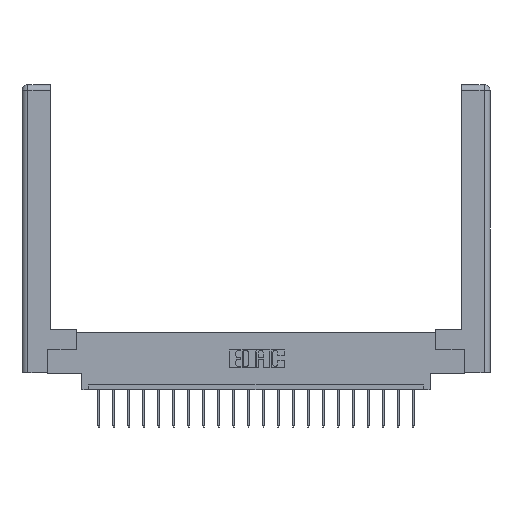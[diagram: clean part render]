
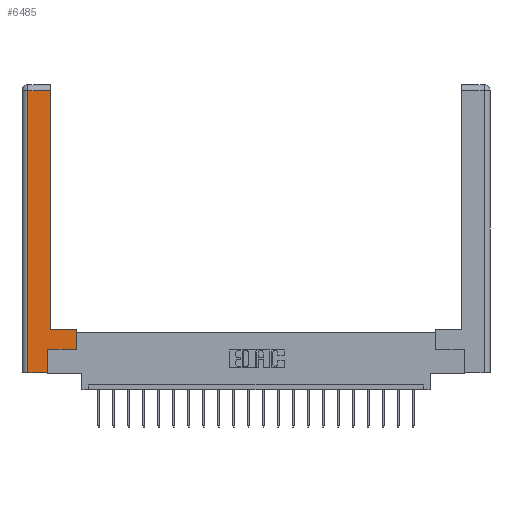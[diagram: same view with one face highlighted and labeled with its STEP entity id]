
A CAD part, top view. The second image highlights one B-rep face of the part: STEP entity #6485.
In plain terms, the highlighted planar face has unit normal (0, 0, 1).
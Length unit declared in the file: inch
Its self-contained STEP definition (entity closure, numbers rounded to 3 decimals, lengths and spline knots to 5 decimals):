
#283 = VERTEX_POINT ( 'NONE', #10952 ) ;
#550 = CARTESIAN_POINT ( 'NONE',  ( 0.0615, 0., 0. ) ) ;
#980 = CARTESIAN_POINT ( 'NONE',  ( 0.565, 0.45, 0. ) ) ;
#1034 = EDGE_CURVE ( 'NONE', #2559, #15257, #3700, .T. ) ;
#1696 = ORIENTED_EDGE ( 'NONE', *, *, #19010, .T. ) ;
#1902 = EDGE_CURVE ( 'NONE', #12222, #6692, #17325, .T. ) ;
#2559 = VERTEX_POINT ( 'NONE', #18048 ) ;
#2889 = VECTOR ( 'NONE', #8444, 39.37008 ) ;
#3086 = DIRECTION ( 'NONE',  ( 0., 0., -1. ) ) ;
#3100 = CARTESIAN_POINT ( 'NONE',  ( 0.295, 0.45, 0. ) ) ;
#3181 = CARTESIAN_POINT ( 'NONE',  ( 0.295, 2.94, 0. ) ) ;
#3634 = FACE_OUTER_BOUND ( 'NONE', #5807, .T. ) ;
#3700 = LINE ( 'NONE', #15891, #17621 ) ;
#4054 = ORIENTED_EDGE ( 'NONE', *, *, #15213, .T. ) ;
#4450 = VECTOR ( 'NONE', #7974, 39.37008 ) ;
#4547 = CARTESIAN_POINT ( 'NONE',  ( 0.565, 0.245, 0. ) ) ;
#5807 = EDGE_LOOP ( 'NONE', ( #4054, #19135, #12590, #9939, #9728, #1696, #17788, #13337 ) ) ;
#6485 = ADVANCED_FACE ( 'NONE', ( #3634 ), #11439, .F. ) ;
#6692 = VERTEX_POINT ( 'NONE', #550 ) ;
#7974 = DIRECTION ( 'NONE',  ( 1., 0., 0. ) ) ;
#8112 = VERTEX_POINT ( 'NONE', #3100 ) ;
#8289 = LINE ( 'NONE', #17586, #18035 ) ;
#8444 = DIRECTION ( 'NONE',  ( 0., -1., 0. ) ) ;
#8876 = LINE ( 'NONE', #4547, #4450 ) ;
#9175 = EDGE_CURVE ( 'NONE', #13286, #283, #17426, .T. ) ;
#9404 = VECTOR ( 'NONE', #20173, 39.37008 ) ;
#9728 = ORIENTED_EDGE ( 'NONE', *, *, #1034, .T. ) ;
#9811 = DIRECTION ( 'NONE',  ( -1., 0., 0. ) ) ;
#9939 = ORIENTED_EDGE ( 'NONE', *, *, #19619, .T. ) ;
#10952 = CARTESIAN_POINT ( 'NONE',  ( 0.565, 0.45, 0. ) ) ;
#11193 = DIRECTION ( 'NONE',  ( 0., 1., 0. ) ) ;
#11387 = DIRECTION ( 'NONE',  ( -1., 0., 0. ) ) ;
#11439 = PLANE ( 'NONE',  #18159 ) ;
#12222 = VERTEX_POINT ( 'NONE', #15771 ) ;
#12590 = ORIENTED_EDGE ( 'NONE', *, *, #1902, .T. ) ;
#12798 = LINE ( 'NONE', #13486, #9404 ) ;
#13012 = EDGE_CURVE ( 'NONE', #13181, #12222, #20869, .T. ) ;
#13027 = CARTESIAN_POINT ( 'NONE',  ( 0., 0., 0. ) ) ;
#13181 = VERTEX_POINT ( 'NONE', #3181 ) ;
#13286 = VERTEX_POINT ( 'NONE', #18941 ) ;
#13337 = ORIENTED_EDGE ( 'NONE', *, *, #15268, .T. ) ;
#13486 = CARTESIAN_POINT ( 'NONE',  ( 0.265, 0., 0. ) ) ;
#14072 = LINE ( 'NONE', #14487, #21687 ) ;
#14261 = DIRECTION ( 'NONE',  ( -1., 0., 0. ) ) ;
#14487 = CARTESIAN_POINT ( 'NONE',  ( 0.295, 3., 0. ) ) ;
#14568 = CARTESIAN_POINT ( 'NONE',  ( 0.265, 0.245, 0. ) ) ;
#15208 = CARTESIAN_POINT ( 'NONE',  ( 0.0615, 2.94, 0. ) ) ;
#15213 = EDGE_CURVE ( 'NONE', #8112, #13181, #14072, .T. ) ;
#15257 = VERTEX_POINT ( 'NONE', #14568 ) ;
#15268 = EDGE_CURVE ( 'NONE', #283, #8112, #8289, .T. ) ;
#15737 = DIRECTION ( 'NONE',  ( 0., 1., 0. ) ) ;
#15755 = CARTESIAN_POINT ( 'NONE',  ( 0.0615, 0., 0. ) ) ;
#15771 = CARTESIAN_POINT ( 'NONE',  ( 0.0615, 2.94, 0. ) ) ;
#15891 = CARTESIAN_POINT ( 'NONE',  ( 0.265, 0.245, 0. ) ) ;
#16892 = VECTOR ( 'NONE', #15737, 39.37008 ) ;
#17325 = LINE ( 'NONE', #15755, #2889 ) ;
#17426 = LINE ( 'NONE', #980, #16892 ) ;
#17586 = CARTESIAN_POINT ( 'NONE',  ( 0.295, 0.45, 0. ) ) ;
#17621 = VECTOR ( 'NONE', #19348, 39.37008 ) ;
#17788 = ORIENTED_EDGE ( 'NONE', *, *, #9175, .T. ) ;
#18035 = VECTOR ( 'NONE', #14261, 39.37008 ) ;
#18048 = CARTESIAN_POINT ( 'NONE',  ( 0.265, 0., 0. ) ) ;
#18159 = AXIS2_PLACEMENT_3D ( 'NONE', #13027, #3086, #9811 ) ;
#18777 = VECTOR ( 'NONE', #11387, 39.37008 ) ;
#18941 = CARTESIAN_POINT ( 'NONE',  ( 0.565, 0.245, 0. ) ) ;
#19010 = EDGE_CURVE ( 'NONE', #15257, #13286, #8876, .T. ) ;
#19135 = ORIENTED_EDGE ( 'NONE', *, *, #13012, .T. ) ;
#19348 = DIRECTION ( 'NONE',  ( 0., 1., 0. ) ) ;
#19619 = EDGE_CURVE ( 'NONE', #6692, #2559, #12798, .T. ) ;
#20173 = DIRECTION ( 'NONE',  ( 1., 0., 0. ) ) ;
#20869 = LINE ( 'NONE', #15208, #18777 ) ;
#21687 = VECTOR ( 'NONE', #11193, 39.37008 ) ;
